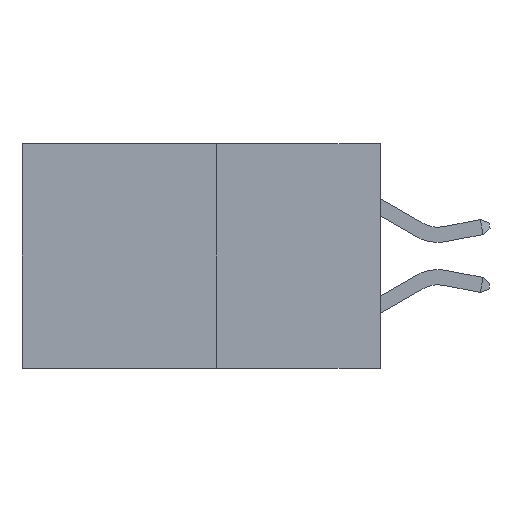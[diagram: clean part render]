
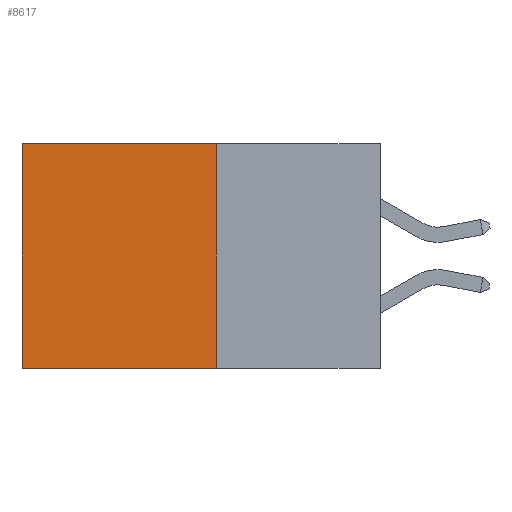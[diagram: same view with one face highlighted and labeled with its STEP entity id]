
A CAD part, left-side view. The second image highlights one B-rep face of the part: STEP entity #8617.
In plain terms, the highlighted planar face has unit normal (-1, 0, 0).
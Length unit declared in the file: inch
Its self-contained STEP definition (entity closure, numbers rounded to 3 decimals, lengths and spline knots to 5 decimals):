
#1043 = DIRECTION ( 'NONE',  ( 0., 0., -1. ) ) ;
#1393 = EDGE_CURVE ( 'NONE', #4172, #11462, #5823, .T. ) ;
#1904 = ORIENTED_EDGE ( 'NONE', *, *, #1393, .F. ) ;
#2331 = LINE ( 'NONE', #12449, #7209 ) ;
#2871 = CARTESIAN_POINT ( 'NONE',  ( 0.277, 0.27, -0.37 ) ) ;
#3000 = LINE ( 'NONE', #3887, #8164 ) ;
#3433 = FACE_OUTER_BOUND ( 'NONE', #11374, .T. ) ;
#3887 = CARTESIAN_POINT ( 'NONE',  ( 0.277, 0.27, 0. ) ) ;
#3948 = EDGE_CURVE ( 'NONE', #4172, #5124, #3000, .T. ) ;
#4172 = VERTEX_POINT ( 'NONE', #6363 ) ;
#4215 = CARTESIAN_POINT ( 'NONE',  ( 0.277, 0.59, -0.37 ) ) ;
#4566 = ORIENTED_EDGE ( 'NONE', *, *, #12426, .T. ) ;
#5048 = PLANE ( 'NONE',  #12854 ) ;
#5124 = VERTEX_POINT ( 'NONE', #10773 ) ;
#5129 = CARTESIAN_POINT ( 'NONE',  ( 0.277, 0.27, -0.37 ) ) ;
#5229 = DIRECTION ( 'NONE',  ( 0., 1., 0. ) ) ;
#5823 = LINE ( 'NONE', #5129, #10623 ) ;
#6076 = DIRECTION ( 'NONE',  ( 1., 0., 0. ) ) ;
#6363 = CARTESIAN_POINT ( 'NONE',  ( 0.277, 0.27, 0. ) ) ;
#6853 = CARTESIAN_POINT ( 'NONE',  ( 0.277, 0.27, -0.37 ) ) ;
#7209 = VECTOR ( 'NONE', #10458, 39.37008 ) ;
#7941 = EDGE_CURVE ( 'NONE', #11462, #12891, #11137, .T. ) ;
#8107 = VECTOR ( 'NONE', #11897, 39.37008 ) ;
#8164 = VECTOR ( 'NONE', #5229, 39.37008 ) ;
#8617 = ADVANCED_FACE ( 'NONE', ( #3433 ), #5048, .F. ) ;
#10458 = DIRECTION ( 'NONE',  ( 0., 0., -1. ) ) ;
#10623 = VECTOR ( 'NONE', #1043, 39.37008 ) ;
#10773 = CARTESIAN_POINT ( 'NONE',  ( 0.277, 0.59, 0. ) ) ;
#10964 = ORIENTED_EDGE ( 'NONE', *, *, #7941, .F. ) ;
#10995 = CARTESIAN_POINT ( 'NONE',  ( 0.277, 0.27, -0.37 ) ) ;
#11120 = ORIENTED_EDGE ( 'NONE', *, *, #3948, .T. ) ;
#11137 = LINE ( 'NONE', #6853, #8107 ) ;
#11374 = EDGE_LOOP ( 'NONE', ( #4566, #10964, #1904, #11120 ) ) ;
#11462 = VERTEX_POINT ( 'NONE', #10995 ) ;
#11897 = DIRECTION ( 'NONE',  ( 0., 1., 0. ) ) ;
#12426 = EDGE_CURVE ( 'NONE', #5124, #12891, #2331, .T. ) ;
#12449 = CARTESIAN_POINT ( 'NONE',  ( 0.277, 0.59, -0.37 ) ) ;
#12854 = AXIS2_PLACEMENT_3D ( 'NONE', #2871, #6076, #13144 ) ;
#12891 = VERTEX_POINT ( 'NONE', #4215 ) ;
#13144 = DIRECTION ( 'NONE',  ( 0., 0., -1. ) ) ;
